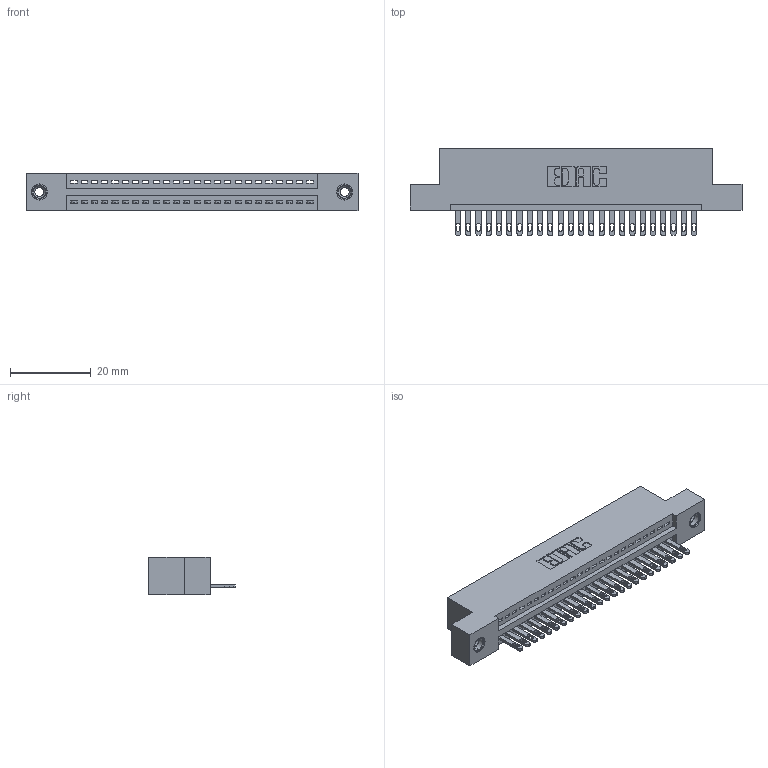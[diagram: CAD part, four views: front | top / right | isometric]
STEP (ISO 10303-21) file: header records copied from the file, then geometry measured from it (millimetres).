
FILE_DESCRIPTION (( 'STEP AP203' ), '1' );
FILE_NAME ('345-024-500-108.STEP', '2018-08-21T04:17:45', ( '' ), ( '' ), 'SwSTEP 2.0', 'SolidWorks 2016', '' );
FILE_SCHEMA (( 'CONFIG_CONTROL_DESIGN' ));
Length unit declared in the file: inch
Products named in the file (4): 345-024-500-108; 345 Part_Flush Mounting Lugs - 0.156 Dia-TI; 345-292-001_345-293-100; 345-250-001_345-250-003-102
Assembly tree (27 placements, depth 2):
  345-024-500-108
    345 Part_Flush Mounting Lugs - 0.156 Dia-TI
    345-292-001_345-293-100  x24
    345-250-001_345-250-003-102  x2
Bounding box: 82.17 x 21.51 x 9.4 mm (x, y, z)
Volume: 7665.4 mm3; surface area: 10015 mm2
Topology: 27 solids, 27 shells, 1482 faces, 4509 edges, 2998 vertices
Faces by surface type: plane 928, cylinder 538, cone 12, torus 4
Entity records: 21602 total; most frequent: CARTESIAN_POINT 3723, ORIENTED_EDGE 3674, DIRECTION 3307, EDGE_CURVE 1837, VECTOR 1585, LINE 1585, VERTEX_POINT 1220, AXIS2_PLACEMENT_3D 861
